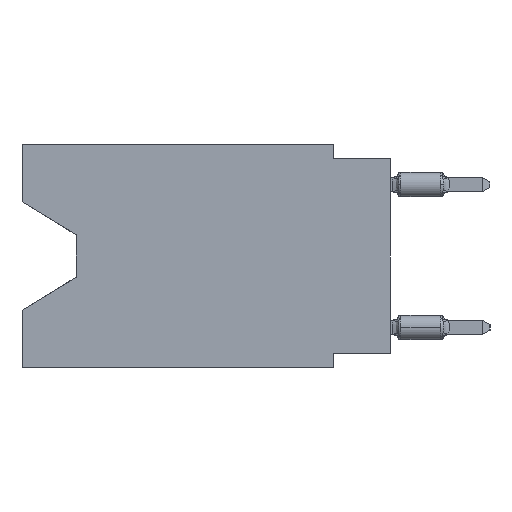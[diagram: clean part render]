
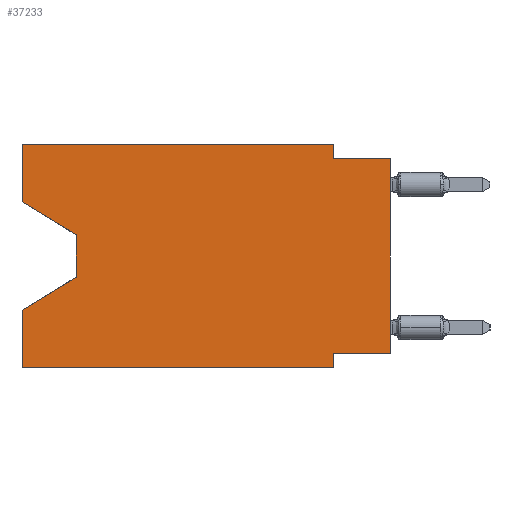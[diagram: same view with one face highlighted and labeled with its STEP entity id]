
A CAD part, left-side view. The second image highlights one B-rep face of the part: STEP entity #37233.
In plain terms, the highlighted planar face has unit normal (-1, 0, 0).
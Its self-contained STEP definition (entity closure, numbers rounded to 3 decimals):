
#396 = EDGE_CURVE ( 'NONE', #14633, #9729, #8385, .T. ) ;
#1016 = ORIENTED_EDGE ( 'NONE', *, *, #15016, .F. ) ;
#1285 = CARTESIAN_POINT ( 'NONE',  ( 0., 13.97, -5.893 ) ) ;
#2203 = VERTEX_POINT ( 'NONE', #6195 ) ;
#2316 = CARTESIAN_POINT ( 'NONE',  ( 0., 0., -9.271 ) ) ;
#2503 = EDGE_CURVE ( 'NONE', #36061, #13265, #4974, .T. ) ;
#2870 = VERTEX_POINT ( 'NONE', #38369 ) ;
#2964 = ORIENTED_EDGE ( 'NONE', *, *, #36396, .T. ) ;
#3798 = LINE ( 'NONE', #4005, #11039 ) ;
#4005 = CARTESIAN_POINT ( 'NONE',  ( 0., 0., 0. ) ) ;
#4181 = CARTESIAN_POINT ( 'NONE',  ( 0., 2.54, 0. ) ) ;
#4625 = CARTESIAN_POINT ( 'NONE',  ( 0., 2.54, -9.271 ) ) ;
#4849 = VECTOR ( 'NONE', #15072, 1000. ) ;
#4974 = LINE ( 'NONE', #19814, #7896 ) ;
#5162 = CARTESIAN_POINT ( 'NONE',  ( 0., 16.383, -9.906 ) ) ;
#5407 = CARTESIAN_POINT ( 'NONE',  ( 0., 16.383, 0. ) ) ;
#5608 = DIRECTION ( 'NONE',  ( 0., 0., 1. ) ) ;
#5705 = EDGE_CURVE ( 'NONE', #9729, #2203, #17839, .T. ) ;
#5877 = VECTOR ( 'NONE', #12225, 1000. ) ;
#6195 = CARTESIAN_POINT ( 'NONE',  ( 0., 2.54, -0.635 ) ) ;
#6981 = VERTEX_POINT ( 'NONE', #13393 ) ;
#7021 = DIRECTION ( 'NONE',  ( 0., 0., 1. ) ) ;
#7726 = DIRECTION ( 'NONE',  ( 0., 0., 1. ) ) ;
#7768 = VERTEX_POINT ( 'NONE', #4625 ) ;
#7896 = VECTOR ( 'NONE', #35207, 1000. ) ;
#8205 = LINE ( 'NONE', #8795, #19728 ) ;
#8385 = LINE ( 'NONE', #17381, #12891 ) ;
#8575 = DIRECTION ( 'NONE',  ( 0., -1., 0. ) ) ;
#8795 = CARTESIAN_POINT ( 'NONE',  ( 0., 0., -0.635 ) ) ;
#8851 = VECTOR ( 'NONE', #32857, 1000. ) ;
#9194 = VECTOR ( 'NONE', #5608, 1000. ) ;
#9729 = VERTEX_POINT ( 'NONE', #4181 ) ;
#11039 = VECTOR ( 'NONE', #7021, 1000. ) ;
#11081 = CARTESIAN_POINT ( 'NONE',  ( 0., 16.383, 0. ) ) ;
#11170 = LINE ( 'NONE', #5162, #25458 ) ;
#11216 = LINE ( 'NONE', #5407, #9194 ) ;
#11287 = CARTESIAN_POINT ( 'NONE',  ( 0., 16.383, 0. ) ) ;
#12011 = ORIENTED_EDGE ( 'NONE', *, *, #5705, .F. ) ;
#12021 = CARTESIAN_POINT ( 'NONE',  ( 0., 0., -9.271 ) ) ;
#12225 = DIRECTION ( 'NONE',  ( 0., 1., 0. ) ) ;
#12260 = CARTESIAN_POINT ( 'NONE',  ( 0., 2.54, -9.906 ) ) ;
#12891 = VECTOR ( 'NONE', #8575, 1000. ) ;
#12955 = CARTESIAN_POINT ( 'NONE',  ( 0., 13.97, -5.893 ) ) ;
#13265 = VERTEX_POINT ( 'NONE', #1285 ) ;
#13393 = CARTESIAN_POINT ( 'NONE',  ( 0., 16.383, -9.906 ) ) ;
#13904 = EDGE_CURVE ( 'NONE', #26340, #7768, #39456, .T. ) ;
#14633 = VERTEX_POINT ( 'NONE', #20839 ) ;
#14985 = DIRECTION ( 'NONE',  ( 0., -1., 0. ) ) ;
#15016 = EDGE_CURVE ( 'NONE', #2203, #15805, #8205, .T. ) ;
#15072 = DIRECTION ( 'NONE',  ( 0., -0.855, -0.519 ) ) ;
#15480 = CARTESIAN_POINT ( 'NONE',  ( 0., 16.383, -2.546 ) ) ;
#15805 = VERTEX_POINT ( 'NONE', #35500 ) ;
#16547 = VECTOR ( 'NONE', #7726, 1000. ) ;
#16556 = ORIENTED_EDGE ( 'NONE', *, *, #31492, .F. ) ;
#16848 = CARTESIAN_POINT ( 'NONE',  ( 0., 16.383, -2.546 ) ) ;
#17296 = PLANE ( 'NONE',  #35691 ) ;
#17381 = CARTESIAN_POINT ( 'NONE',  ( 0., 16.383, 0. ) ) ;
#17445 = CARTESIAN_POINT ( 'NONE',  ( 0., 2.54, 0. ) ) ;
#17839 = LINE ( 'NONE', #17445, #21781 ) ;
#18143 = ORIENTED_EDGE ( 'NONE', *, *, #13904, .F. ) ;
#18685 = LINE ( 'NONE', #15480, #4849 ) ;
#18768 = ORIENTED_EDGE ( 'NONE', *, *, #21023, .T. ) ;
#19713 = DIRECTION ( 'NONE',  ( 0., 0., -1. ) ) ;
#19728 = VECTOR ( 'NONE', #14985, 1000. ) ;
#19789 = EDGE_CURVE ( 'NONE', #22183, #36061, #18685, .T. ) ;
#19814 = CARTESIAN_POINT ( 'NONE',  ( 0., 13.97, -4.013 ) ) ;
#20581 = DIRECTION ( 'NONE',  ( 0., -1., 0. ) ) ;
#20645 = ORIENTED_EDGE ( 'NONE', *, *, #19789, .T. ) ;
#20839 = CARTESIAN_POINT ( 'NONE',  ( 0., 16.383, 0. ) ) ;
#21023 = EDGE_CURVE ( 'NONE', #26340, #15805, #3798, .T. ) ;
#21781 = VECTOR ( 'NONE', #32226, 1000. ) ;
#22167 = DIRECTION ( 'NONE',  ( 0., 0.855, -0.519 ) ) ;
#22183 = VERTEX_POINT ( 'NONE', #16848 ) ;
#22353 = EDGE_CURVE ( 'NONE', #22183, #14633, #11216, .T. ) ;
#22567 = LINE ( 'NONE', #12955, #36294 ) ;
#23285 = FACE_OUTER_BOUND ( 'NONE', #34233, .T. ) ;
#25458 = VECTOR ( 'NONE', #20581, 1000. ) ;
#26340 = VERTEX_POINT ( 'NONE', #2316 ) ;
#27866 = ORIENTED_EDGE ( 'NONE', *, *, #396, .F. ) ;
#28555 = ORIENTED_EDGE ( 'NONE', *, *, #2503, .T. ) ;
#30031 = VERTEX_POINT ( 'NONE', #30911 ) ;
#30373 = ORIENTED_EDGE ( 'NONE', *, *, #22353, .F. ) ;
#30675 = ORIENTED_EDGE ( 'NONE', *, *, #38472, .F. ) ;
#30868 = EDGE_CURVE ( 'NONE', #13265, #30031, #22567, .T. ) ;
#30911 = CARTESIAN_POINT ( 'NONE',  ( 0., 16.383, -7.36 ) ) ;
#31492 = EDGE_CURVE ( 'NONE', #7768, #2870, #35885, .T. ) ;
#32226 = DIRECTION ( 'NONE',  ( 0., 0., -1. ) ) ;
#32457 = CARTESIAN_POINT ( 'NONE',  ( 0., 13.97, -4.013 ) ) ;
#32857 = DIRECTION ( 'NONE',  ( 0., 0., -1. ) ) ;
#34233 = EDGE_LOOP ( 'NONE', ( #20645, #28555, #35568, #30675, #2964, #16556, #18143, #18768, #1016, #12011, #27866, #30373 ) ) ;
#35207 = DIRECTION ( 'NONE',  ( 0., 0., -1. ) ) ;
#35486 = DIRECTION ( 'NONE',  ( 1., 0., 0. ) ) ;
#35494 = LINE ( 'NONE', #11287, #16547 ) ;
#35500 = CARTESIAN_POINT ( 'NONE',  ( 0., 0., -0.635 ) ) ;
#35568 = ORIENTED_EDGE ( 'NONE', *, *, #30868, .T. ) ;
#35691 = AXIS2_PLACEMENT_3D ( 'NONE', #11081, #35486, #19713 ) ;
#35885 = LINE ( 'NONE', #12260, #8851 ) ;
#36061 = VERTEX_POINT ( 'NONE', #32457 ) ;
#36294 = VECTOR ( 'NONE', #22167, 1000. ) ;
#36396 = EDGE_CURVE ( 'NONE', #6981, #2870, #11170, .T. ) ;
#37233 = ADVANCED_FACE ( 'NONE', ( #23285 ), #17296, .F. ) ;
#38369 = CARTESIAN_POINT ( 'NONE',  ( 0., 2.54, -9.906 ) ) ;
#38472 = EDGE_CURVE ( 'NONE', #6981, #30031, #35494, .T. ) ;
#39456 = LINE ( 'NONE', #12021, #5877 ) ;
